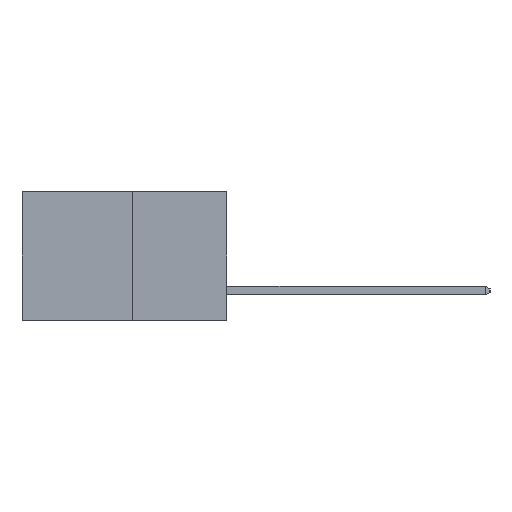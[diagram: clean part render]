
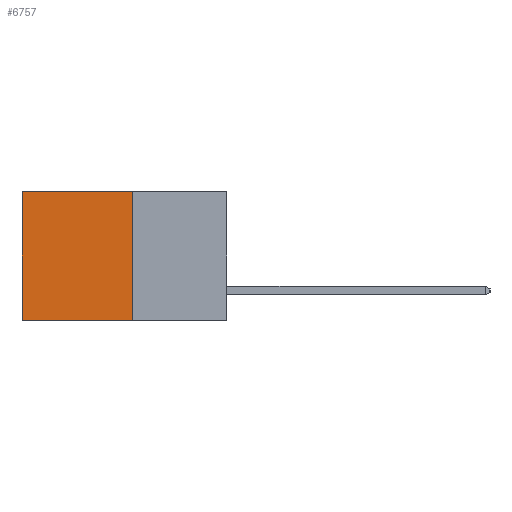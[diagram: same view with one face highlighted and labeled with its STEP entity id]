
A CAD part, left-side view. The second image highlights one B-rep face of the part: STEP entity #6757.
In plain terms, the highlighted planar face has unit normal (-1, 0, 0).
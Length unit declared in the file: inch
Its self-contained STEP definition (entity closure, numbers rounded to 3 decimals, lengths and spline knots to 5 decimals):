
#94 = DIRECTION ( 'NONE',  ( 0., 1., 0. ) ) ;
#364 = CARTESIAN_POINT ( 'NONE',  ( 0.277, 0.27, 0. ) ) ;
#377 = EDGE_LOOP ( 'NONE', ( #7799, #7794, #8046, #8098 ) ) ;
#465 = VECTOR ( 'NONE', #7838, 39.37008 ) ;
#787 = EDGE_CURVE ( 'NONE', #7436, #5229, #5530, .T. ) ;
#910 = FACE_OUTER_BOUND ( 'NONE', #377, .T. ) ;
#1053 = VECTOR ( 'NONE', #7012, 39.37008 ) ;
#1882 = CARTESIAN_POINT ( 'NONE',  ( 0.277, 0.27, -0.37 ) ) ;
#2309 = CARTESIAN_POINT ( 'NONE',  ( 0.277, 0.27, -0.37 ) ) ;
#3415 = CARTESIAN_POINT ( 'NONE',  ( 0.277, 0.27, 0. ) ) ;
#3622 = CARTESIAN_POINT ( 'NONE',  ( 0.277, 0.59, 0. ) ) ;
#4011 = VERTEX_POINT ( 'NONE', #3415 ) ;
#4348 = EDGE_CURVE ( 'NONE', #4011, #7436, #7690, .T. ) ;
#4629 = AXIS2_PLACEMENT_3D ( 'NONE', #8030, #7886, #7875 ) ;
#4884 = LINE ( 'NONE', #7196, #465 ) ;
#5229 = VERTEX_POINT ( 'NONE', #7869 ) ;
#5346 = LINE ( 'NONE', #364, #1053 ) ;
#5495 = EDGE_CURVE ( 'NONE', #4011, #8927, #5346, .T. ) ;
#5530 = LINE ( 'NONE', #1882, #7744 ) ;
#6757 = ADVANCED_FACE ( 'NONE', ( #910 ), #7969, .F. ) ;
#7012 = DIRECTION ( 'NONE',  ( 0., 1., 0. ) ) ;
#7196 = CARTESIAN_POINT ( 'NONE',  ( 0.277, 0.59, -0.37 ) ) ;
#7436 = VERTEX_POINT ( 'NONE', #2309 ) ;
#7690 = LINE ( 'NONE', #9330, #9282 ) ;
#7744 = VECTOR ( 'NONE', #94, 39.37008 ) ;
#7794 = ORIENTED_EDGE ( 'NONE', *, *, #787, .F. ) ;
#7799 = ORIENTED_EDGE ( 'NONE', *, *, #8950, .T. ) ;
#7838 = DIRECTION ( 'NONE',  ( 0., 0., -1. ) ) ;
#7869 = CARTESIAN_POINT ( 'NONE',  ( 0.277, 0.59, -0.37 ) ) ;
#7875 = DIRECTION ( 'NONE',  ( 0., 0., -1. ) ) ;
#7886 = DIRECTION ( 'NONE',  ( 1., 0., 0. ) ) ;
#7969 = PLANE ( 'NONE',  #4629 ) ;
#8030 = CARTESIAN_POINT ( 'NONE',  ( 0.277, 0.27, -0.37 ) ) ;
#8046 = ORIENTED_EDGE ( 'NONE', *, *, #4348, .F. ) ;
#8098 = ORIENTED_EDGE ( 'NONE', *, *, #5495, .T. ) ;
#8619 = DIRECTION ( 'NONE',  ( 0., 0., -1. ) ) ;
#8927 = VERTEX_POINT ( 'NONE', #3622 ) ;
#8950 = EDGE_CURVE ( 'NONE', #8927, #5229, #4884, .T. ) ;
#9282 = VECTOR ( 'NONE', #8619, 39.37008 ) ;
#9330 = CARTESIAN_POINT ( 'NONE',  ( 0.277, 0.27, -0.37 ) ) ;
